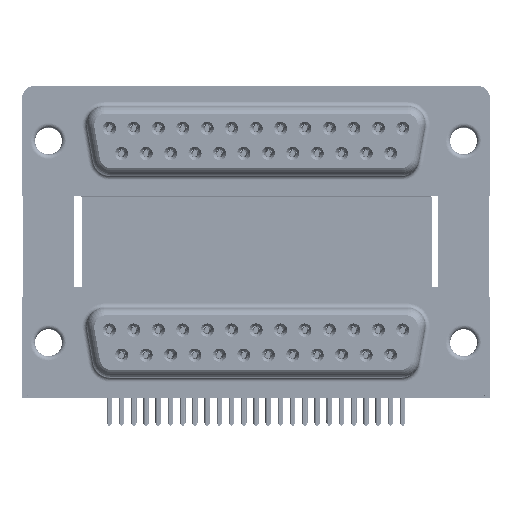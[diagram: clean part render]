
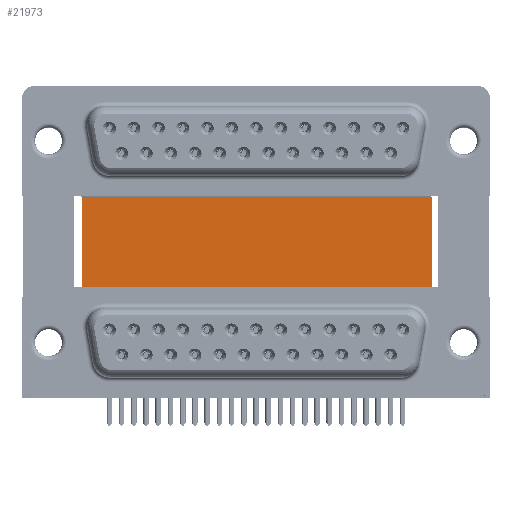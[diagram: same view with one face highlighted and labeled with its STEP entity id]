
A CAD part, top view. The second image highlights one B-rep face of the part: STEP entity #21973.
In plain terms, the highlighted planar face has unit normal (0, 0, 1).
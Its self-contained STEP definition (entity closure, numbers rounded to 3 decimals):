
#2397 = DIRECTION ( 'NONE',  ( -1., 0., 0. ) ) ;
#3301 = DIRECTION ( 'NONE',  ( 0., 0., -1. ) ) ;
#4713 = EDGE_CURVE ( 'NONE', #21018, #4980, #27787, .T. ) ;
#4980 = VERTEX_POINT ( 'NONE', #27124 ) ;
#6571 = LINE ( 'NONE', #16690, #43849 ) ;
#6705 = CARTESIAN_POINT ( 'NONE',  ( 3.79, 16.585, -12. ) ) ;
#6990 = VECTOR ( 'NONE', #51615, 1000. ) ;
#10878 = VERTEX_POINT ( 'NONE', #23937 ) ;
#14993 = ORIENTED_EDGE ( 'NONE', *, *, #34507, .T. ) ;
#16690 = CARTESIAN_POINT ( 'NONE',  ( 3.79, 16.585, -12. ) ) ;
#17752 = ORIENTED_EDGE ( 'NONE', *, *, #34671, .T. ) ;
#21018 = VERTEX_POINT ( 'NONE', #35348 ) ;
#21973 = ADVANCED_FACE ( 'NONE', ( #34839 ), #49800, .F. ) ;
#23937 = CARTESIAN_POINT ( 'NONE',  ( 3.79, -3.735, -12. ) ) ;
#25220 = DIRECTION ( 'NONE',  ( 0., -1., 0. ) ) ;
#26867 = ORIENTED_EDGE ( 'NONE', *, *, #36860, .F. ) ;
#27124 = CARTESIAN_POINT ( 'NONE',  ( 43.43, 16.585, -12. ) ) ;
#27787 = LINE ( 'NONE', #33257, #6990 ) ;
#28304 = LINE ( 'NONE', #46942, #53589 ) ;
#31313 = VECTOR ( 'NONE', #36051, 1000. ) ;
#32400 = CARTESIAN_POINT ( 'NONE',  ( 43.43, -3.735, -12. ) ) ;
#33257 = CARTESIAN_POINT ( 'NONE',  ( 3.79, 16.585, -12. ) ) ;
#34507 = EDGE_CURVE ( 'NONE', #10878, #60134, #28304, .T. ) ;
#34671 = EDGE_CURVE ( 'NONE', #21018, #10878, #6571, .T. ) ;
#34839 = FACE_OUTER_BOUND ( 'NONE', #47445, .T. ) ;
#35348 = CARTESIAN_POINT ( 'NONE',  ( 3.79, 16.585, -12. ) ) ;
#36051 = DIRECTION ( 'NONE',  ( 0., -1., 0. ) ) ;
#36192 = AXIS2_PLACEMENT_3D ( 'NONE', #6705, #3301, #2397 ) ;
#36860 = EDGE_CURVE ( 'NONE', #4980, #60134, #59650, .T. ) ;
#38308 = ORIENTED_EDGE ( 'NONE', *, *, #4713, .F. ) ;
#42336 = DIRECTION ( 'NONE',  ( 1., 0., 0. ) ) ;
#43849 = VECTOR ( 'NONE', #25220, 1000. ) ;
#46942 = CARTESIAN_POINT ( 'NONE',  ( 3.79, -3.735, -12. ) ) ;
#47445 = EDGE_LOOP ( 'NONE', ( #14993, #26867, #38308, #17752 ) ) ;
#49800 = PLANE ( 'NONE',  #36192 ) ;
#51615 = DIRECTION ( 'NONE',  ( 1., 0., 0. ) ) ;
#53589 = VECTOR ( 'NONE', #42336, 1000. ) ;
#54163 = CARTESIAN_POINT ( 'NONE',  ( 43.43, 16.585, -12. ) ) ;
#59650 = LINE ( 'NONE', #54163, #31313 ) ;
#60134 = VERTEX_POINT ( 'NONE', #32400 ) ;
